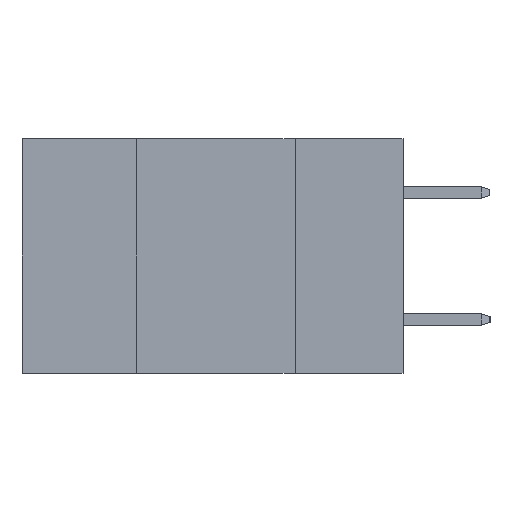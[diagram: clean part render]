
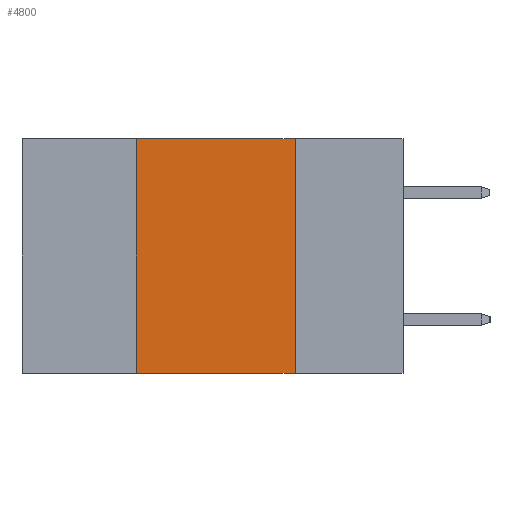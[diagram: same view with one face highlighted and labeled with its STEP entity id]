
A CAD part, left-side view. The second image highlights one B-rep face of the part: STEP entity #4800.
In plain terms, the highlighted planar face has unit normal (-1, 0, 0).
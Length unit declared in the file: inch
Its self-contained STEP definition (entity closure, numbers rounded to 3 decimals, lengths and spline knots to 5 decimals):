
#129 = LINE ( 'NONE', #3625, #7415 ) ;
#189 = EDGE_CURVE ( 'NONE', #8495, #2993, #129, .T. ) ;
#594 = CARTESIAN_POINT ( 'NONE',  ( 0., 0.17, 0. ) ) ;
#1081 = EDGE_CURVE ( 'NONE', #3746, #5253, #10591, .T. ) ;
#1100 = CARTESIAN_POINT ( 'NONE',  ( 0., 0.6, 0. ) ) ;
#1785 = ORIENTED_EDGE ( 'NONE', *, *, #1081, .F. ) ;
#1870 = AXIS2_PLACEMENT_3D ( 'NONE', #1100, #4320, #1981 ) ;
#1946 = CARTESIAN_POINT ( 'NONE',  ( 0., 0.42, -0.37 ) ) ;
#1981 = DIRECTION ( 'NONE',  ( 0., 0., -1. ) ) ;
#2009 = DIRECTION ( 'NONE',  ( 0., -1., 0. ) ) ;
#2452 = ORIENTED_EDGE ( 'NONE', *, *, #2471, .F. ) ;
#2471 = EDGE_CURVE ( 'NONE', #5253, #2993, #8202, .T. ) ;
#2546 = VECTOR ( 'NONE', #3989, 39.37008 ) ;
#2993 = VERTEX_POINT ( 'NONE', #4081 ) ;
#3081 = DIRECTION ( 'NONE',  ( 0., 0., 1. ) ) ;
#3206 = EDGE_LOOP ( 'NONE', ( #2452, #1785, #3923, #6835 ) ) ;
#3625 = CARTESIAN_POINT ( 'NONE',  ( 0., 0.6, -0.37 ) ) ;
#3746 = VERTEX_POINT ( 'NONE', #5371 ) ;
#3923 = ORIENTED_EDGE ( 'NONE', *, *, #9553, .F. ) ;
#3989 = DIRECTION ( 'NONE',  ( 0., 0., -1. ) ) ;
#4081 = CARTESIAN_POINT ( 'NONE',  ( 0., 0.17, -0.37 ) ) ;
#4320 = DIRECTION ( 'NONE',  ( 1., 0., 0. ) ) ;
#4539 = CARTESIAN_POINT ( 'NONE',  ( 0., 0.6, 0. ) ) ;
#4800 = ADVANCED_FACE ( 'NONE', ( #7710 ), #5147, .F. ) ;
#4955 = CARTESIAN_POINT ( 'NONE',  ( 0., 0.42, 0. ) ) ;
#5084 = CARTESIAN_POINT ( 'NONE',  ( 0., 0.17, 0. ) ) ;
#5147 = PLANE ( 'NONE',  #1870 ) ;
#5253 = VERTEX_POINT ( 'NONE', #5084 ) ;
#5371 = CARTESIAN_POINT ( 'NONE',  ( 0., 0.42, 0. ) ) ;
#5698 = VECTOR ( 'NONE', #3081, 39.37008 ) ;
#5758 = VECTOR ( 'NONE', #10696, 39.37008 ) ;
#5798 = LINE ( 'NONE', #4955, #5698 ) ;
#6835 = ORIENTED_EDGE ( 'NONE', *, *, #189, .T. ) ;
#7415 = VECTOR ( 'NONE', #2009, 39.37008 ) ;
#7710 = FACE_OUTER_BOUND ( 'NONE', #3206, .T. ) ;
#8202 = LINE ( 'NONE', #594, #2546 ) ;
#8495 = VERTEX_POINT ( 'NONE', #1946 ) ;
#9553 = EDGE_CURVE ( 'NONE', #8495, #3746, #5798, .T. ) ;
#10591 = LINE ( 'NONE', #4539, #5758 ) ;
#10696 = DIRECTION ( 'NONE',  ( 0., -1., 0. ) ) ;
